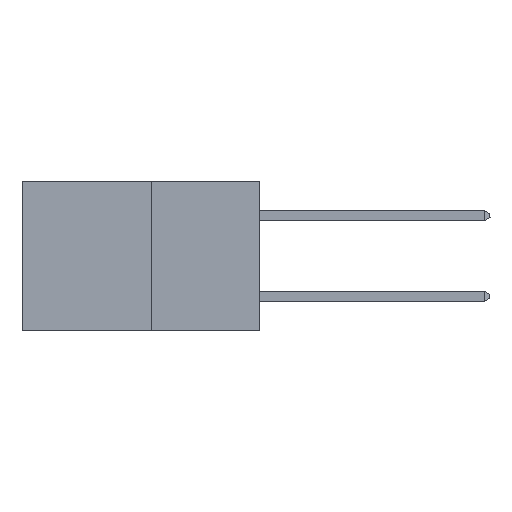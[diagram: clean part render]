
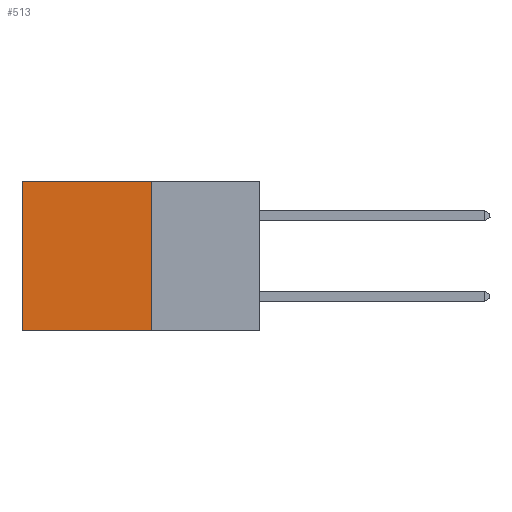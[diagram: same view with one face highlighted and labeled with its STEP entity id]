
A CAD part, left-side view. The second image highlights one B-rep face of the part: STEP entity #513.
In plain terms, the highlighted planar face has unit normal (-1, 0, 0).
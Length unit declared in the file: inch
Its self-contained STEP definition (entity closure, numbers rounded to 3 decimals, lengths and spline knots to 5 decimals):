
#409 = CARTESIAN_POINT ( 'NONE',  ( 0.277, 0.59, 0. ) ) ;
#513 = ADVANCED_FACE ( 'NONE', ( #1311 ), #13749, .F. ) ;
#697 = EDGE_CURVE ( 'NONE', #5273, #1124, #10298, .T. ) ;
#938 = VECTOR ( 'NONE', #4328, 39.37008 ) ;
#1098 = VECTOR ( 'NONE', #2045, 39.37008 ) ;
#1124 = VERTEX_POINT ( 'NONE', #409 ) ;
#1311 = FACE_OUTER_BOUND ( 'NONE', #12722, .T. ) ;
#1324 = LINE ( 'NONE', #4350, #938 ) ;
#1943 = DIRECTION ( 'NONE',  ( 0., 0., -1. ) ) ;
#2045 = DIRECTION ( 'NONE',  ( 0., 1., 0. ) ) ;
#4219 = LINE ( 'NONE', #13441, #9862 ) ;
#4328 = DIRECTION ( 'NONE',  ( 0., 0., -1. ) ) ;
#4350 = CARTESIAN_POINT ( 'NONE',  ( 0.277, 0.59, -0.37 ) ) ;
#4572 = EDGE_CURVE ( 'NONE', #5273, #6435, #4219, .T. ) ;
#4877 = EDGE_CURVE ( 'NONE', #6435, #6006, #8631, .T. ) ;
#5273 = VERTEX_POINT ( 'NONE', #7358 ) ;
#5381 = AXIS2_PLACEMENT_3D ( 'NONE', #8030, #14098, #14094 ) ;
#6006 = VERTEX_POINT ( 'NONE', #6978 ) ;
#6435 = VERTEX_POINT ( 'NONE', #7139 ) ;
#6978 = CARTESIAN_POINT ( 'NONE',  ( 0.277, 0.59, -0.37 ) ) ;
#7139 = CARTESIAN_POINT ( 'NONE',  ( 0.277, 0.27, -0.37 ) ) ;
#7358 = CARTESIAN_POINT ( 'NONE',  ( 0.277, 0.27, 0. ) ) ;
#7393 = EDGE_CURVE ( 'NONE', #1124, #6006, #1324, .T. ) ;
#8030 = CARTESIAN_POINT ( 'NONE',  ( 0.277, 0.27, -0.37 ) ) ;
#8054 = DIRECTION ( 'NONE',  ( 0., 1., 0. ) ) ;
#8514 = CARTESIAN_POINT ( 'NONE',  ( 0.277, 0.27, -0.37 ) ) ;
#8631 = LINE ( 'NONE', #8514, #14069 ) ;
#9862 = VECTOR ( 'NONE', #1943, 39.37008 ) ;
#10298 = LINE ( 'NONE', #12054, #1098 ) ;
#11935 = ORIENTED_EDGE ( 'NONE', *, *, #7393, .T. ) ;
#12032 = ORIENTED_EDGE ( 'NONE', *, *, #4572, .F. ) ;
#12054 = CARTESIAN_POINT ( 'NONE',  ( 0.277, 0.27, 0. ) ) ;
#12262 = ORIENTED_EDGE ( 'NONE', *, *, #4877, .F. ) ;
#12722 = EDGE_LOOP ( 'NONE', ( #11935, #12262, #12032, #14389 ) ) ;
#13441 = CARTESIAN_POINT ( 'NONE',  ( 0.277, 0.27, -0.37 ) ) ;
#13749 = PLANE ( 'NONE',  #5381 ) ;
#14069 = VECTOR ( 'NONE', #8054, 39.37008 ) ;
#14094 = DIRECTION ( 'NONE',  ( 0., 0., -1. ) ) ;
#14098 = DIRECTION ( 'NONE',  ( 1., 0., 0. ) ) ;
#14389 = ORIENTED_EDGE ( 'NONE', *, *, #697, .T. ) ;
